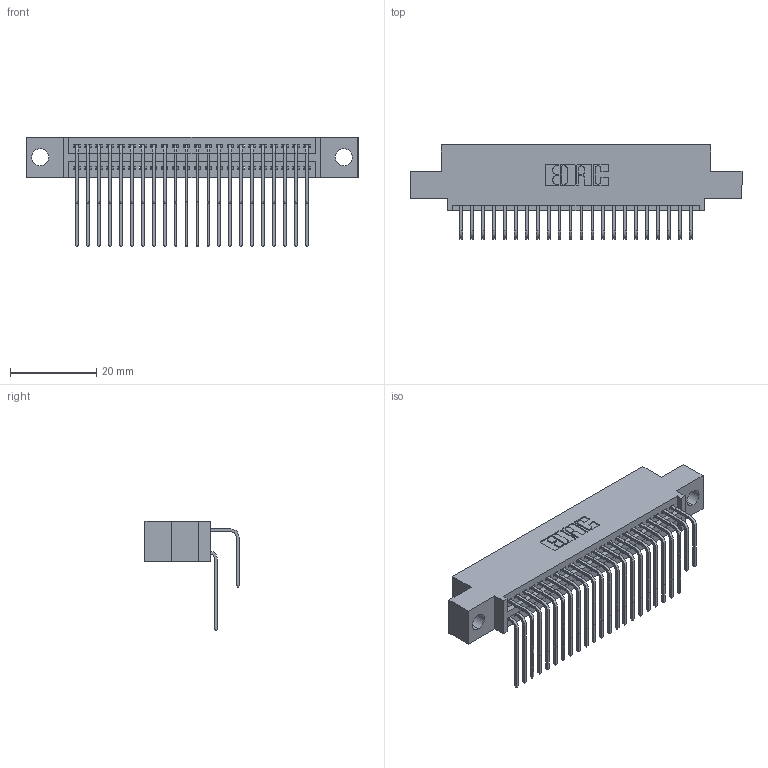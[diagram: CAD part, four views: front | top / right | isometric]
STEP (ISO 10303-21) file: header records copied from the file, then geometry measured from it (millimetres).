
FILE_DESCRIPTION (( 'STEP AP203' ), '1' );
FILE_NAME ('345-044-558-504.STEP', '2021-05-20T02:07:07', ( '' ), ( '' ), 'SwSTEP 2.0', 'SolidWorks 2020', '' );
FILE_SCHEMA (( 'CONFIG_CONTROL_DESIGN' ));
Length unit declared in the file: inch
Products named in the file (4): 345-044-558-504; 345-292-001_558 Tail - 2; 345 Part_0.110 Offset - 0.156 Dia-TI; 345-292-001_558 559 Tail - 1
Assembly tree (45 placements, depth 2):
  345-044-558-504
    345 Part_0.110 Offset - 0.156 Dia-TI
    345-292-001_558 559 Tail - 1  x22
    345-292-001_558 Tail - 2  x22
Bounding box: 77.09 x 21.83 x 25.53 mm (x, y, z)
Volume: 7377.4 mm3; surface area: 11655.6 mm2
Topology: 45 solids, 45 shells, 2432 faces, 7209 edges, 4746 vertices
Faces by surface type: plane 1638, cylinder 794
Entity records: 22157 total; most frequent: CARTESIAN_POINT 3785, ORIENTED_EDGE 3666, DIRECTION 3333, EDGE_CURVE 1833, LINE 1573, VECTOR 1573, VERTEX_POINT 1218, AXIS2_PLACEMENT_3D 880
